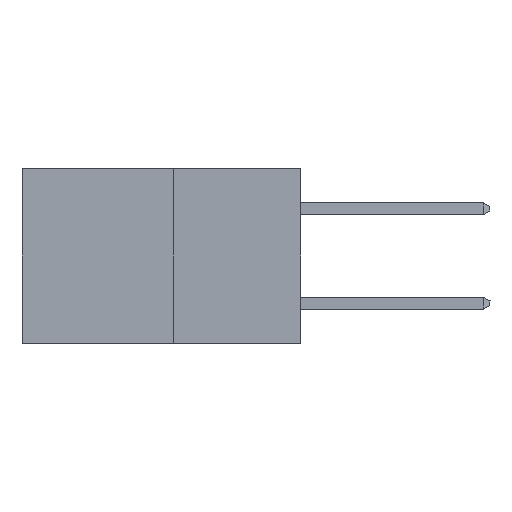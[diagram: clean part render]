
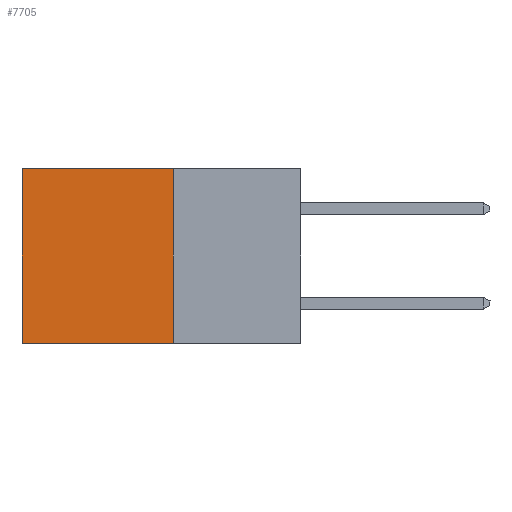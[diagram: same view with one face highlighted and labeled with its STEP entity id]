
A CAD part, left-side view. The second image highlights one B-rep face of the part: STEP entity #7705.
In plain terms, the highlighted planar face has unit normal (-1, 0, 0).
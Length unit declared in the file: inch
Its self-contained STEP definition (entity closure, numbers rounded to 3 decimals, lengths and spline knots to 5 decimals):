
#415 = CARTESIAN_POINT ( 'NONE',  ( 0.277, 0.59, -0.37 ) ) ;
#560 = CARTESIAN_POINT ( 'NONE',  ( 0.277, 0.27, 0. ) ) ;
#1337 = ORIENTED_EDGE ( 'NONE', *, *, #5954, .T. ) ;
#1509 = DIRECTION ( 'NONE',  ( 0., 1., 0. ) ) ;
#1604 = CARTESIAN_POINT ( 'NONE',  ( 0.277, 0.27, -0.37 ) ) ;
#1723 = DIRECTION ( 'NONE',  ( 0., 1., 0. ) ) ;
#2589 = DIRECTION ( 'NONE',  ( 0., 0., -1. ) ) ;
#3408 = CARTESIAN_POINT ( 'NONE',  ( 0.277, 0.59, -0.37 ) ) ;
#4086 = VECTOR ( 'NONE', #12302, 39.37008 ) ;
#4164 = VECTOR ( 'NONE', #1723, 39.37008 ) ;
#4241 = CARTESIAN_POINT ( 'NONE',  ( 0.277, 0.27, -0.37 ) ) ;
#4455 = VERTEX_POINT ( 'NONE', #415 ) ;
#4773 = LINE ( 'NONE', #6636, #4164 ) ;
#5247 = DIRECTION ( 'NONE',  ( 0., 0., -1. ) ) ;
#5935 = EDGE_CURVE ( 'NONE', #9975, #4455, #6732, .T. ) ;
#5954 = EDGE_CURVE ( 'NONE', #7826, #9975, #9408, .T. ) ;
#6148 = ORIENTED_EDGE ( 'NONE', *, *, #5935, .T. ) ;
#6620 = VECTOR ( 'NONE', #2589, 39.37008 ) ;
#6636 = CARTESIAN_POINT ( 'NONE',  ( 0.277, 0.27, -0.37 ) ) ;
#6732 = LINE ( 'NONE', #3408, #4086 ) ;
#6939 = LINE ( 'NONE', #1604, #6620 ) ;
#6987 = CARTESIAN_POINT ( 'NONE',  ( 0.277, 0.27, -0.37 ) ) ;
#7705 = ADVANCED_FACE ( 'NONE', ( #10871 ), #10210, .F. ) ;
#7726 = ORIENTED_EDGE ( 'NONE', *, *, #12025, .F. ) ;
#7826 = VERTEX_POINT ( 'NONE', #9460 ) ;
#7910 = ORIENTED_EDGE ( 'NONE', *, *, #10899, .F. ) ;
#8911 = EDGE_LOOP ( 'NONE', ( #6148, #7910, #7726, #1337 ) ) ;
#9408 = LINE ( 'NONE', #560, #11656 ) ;
#9460 = CARTESIAN_POINT ( 'NONE',  ( 0.277, 0.27, 0. ) ) ;
#9601 = VERTEX_POINT ( 'NONE', #6987 ) ;
#9975 = VERTEX_POINT ( 'NONE', #12640 ) ;
#10210 = PLANE ( 'NONE',  #11368 ) ;
#10871 = FACE_OUTER_BOUND ( 'NONE', #8911, .T. ) ;
#10899 = EDGE_CURVE ( 'NONE', #9601, #4455, #4773, .T. ) ;
#11167 = DIRECTION ( 'NONE',  ( 1., 0., 0. ) ) ;
#11368 = AXIS2_PLACEMENT_3D ( 'NONE', #4241, #11167, #5247 ) ;
#11656 = VECTOR ( 'NONE', #1509, 39.37008 ) ;
#12025 = EDGE_CURVE ( 'NONE', #7826, #9601, #6939, .T. ) ;
#12302 = DIRECTION ( 'NONE',  ( 0., 0., -1. ) ) ;
#12640 = CARTESIAN_POINT ( 'NONE',  ( 0.277, 0.59, 0. ) ) ;
